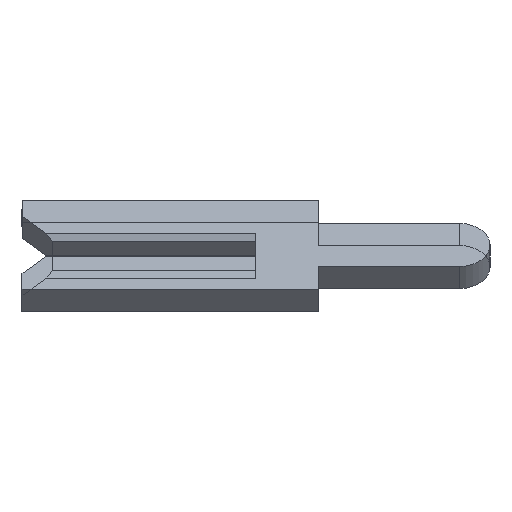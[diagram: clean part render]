
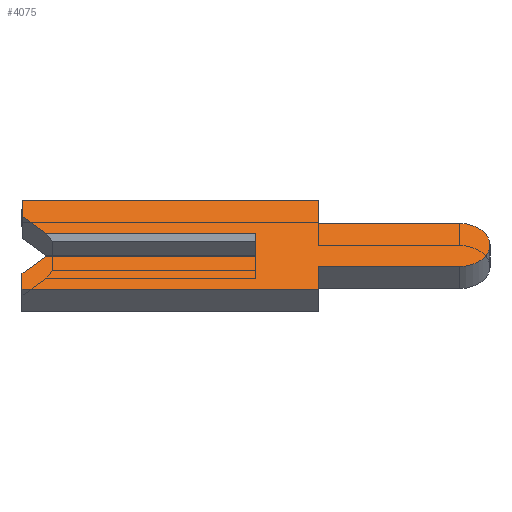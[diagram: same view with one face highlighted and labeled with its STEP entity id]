
A CAD part, left-side view. The second image highlights one B-rep face of the part: STEP entity #4075.
In plain terms, the highlighted face is planar.
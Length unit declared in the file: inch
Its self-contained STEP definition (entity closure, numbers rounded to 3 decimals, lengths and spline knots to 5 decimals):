
#40 = ORIENTED_EDGE ( 'NONE', *, *, #2204, .F. ) ;
#51 = CARTESIAN_POINT ( 'NONE',  ( -0.01, 0., 0.01 ) ) ;
#64 = CARTESIAN_POINT ( 'NONE',  ( -0.01, -0.04, 0.04 ) ) ;
#90 = LINE ( 'NONE', #1590, #3941 ) ;
#174 = VECTOR ( 'NONE', #2166, 39.37008 ) ;
#200 = LINE ( 'NONE', #1992, #308 ) ;
#203 = VERTEX_POINT ( 'NONE', #4058 ) ;
#227 = LINE ( 'NONE', #1441, #3796 ) ;
#308 = VECTOR ( 'NONE', #2768, 39.37008 ) ;
#315 = EDGE_CURVE ( 'NONE', #1802, #699, #2897, .T. ) ;
#431 = CARTESIAN_POINT ( 'NONE',  ( -0.01, 0.15, 0.04 ) ) ;
#466 = EDGE_CURVE ( 'NONE', #2783, #3046, #90, .T. ) ;
#490 = ORIENTED_EDGE ( 'NONE', *, *, #4316, .F. ) ;
#614 = LINE ( 'NONE', #3874, #3076 ) ;
#619 = CARTESIAN_POINT ( 'NONE',  ( -0.01, -0.1305, -0.0195 ) ) ;
#634 = DIRECTION ( 'NONE',  ( 0., 0., -1. ) ) ;
#636 = VERTEX_POINT ( 'NONE', #2024 ) ;
#690 = CARTESIAN_POINT ( 'NONE',  ( -0.01, 0.15, 0.04 ) ) ;
#695 = ORIENTED_EDGE ( 'NONE', *, *, #466, .F. ) ;
#699 = VERTEX_POINT ( 'NONE', #619 ) ;
#790 = PLANE ( 'NONE',  #916 ) ;
#916 = AXIS2_PLACEMENT_3D ( 'NONE', #3235, #1152, #1467 ) ;
#924 = LINE ( 'NONE', #3522, #949 ) ;
#929 = EDGE_LOOP ( 'NONE', ( #932, #3387, #4383, #3278, #1319, #1087, #40, #2142, #2138, #490, #3675, #3049, #695, #1218 ) ) ;
#932 = ORIENTED_EDGE ( 'NONE', *, *, #1268, .T. ) ;
#948 = VECTOR ( 'NONE', #4380, 39.37008 ) ;
#949 = VECTOR ( 'NONE', #2817, 39.37008 ) ;
#1085 = DIRECTION ( 'NONE',  ( 0., 0., 1. ) ) ;
#1087 = ORIENTED_EDGE ( 'NONE', *, *, #1785, .F. ) ;
#1152 = DIRECTION ( 'NONE',  ( 1., 0., 0. ) ) ;
#1169 = CARTESIAN_POINT ( 'NONE',  ( -0.01, -0.04, 0.0195 ) ) ;
#1218 = ORIENTED_EDGE ( 'NONE', *, *, #3611, .F. ) ;
#1268 = EDGE_CURVE ( 'NONE', #3727, #2309, #200, .T. ) ;
#1285 = LINE ( 'NONE', #431, #1708 ) ;
#1289 = LINE ( 'NONE', #4321, #2749 ) ;
#1319 = ORIENTED_EDGE ( 'NONE', *, *, #2436, .F. ) ;
#1441 = CARTESIAN_POINT ( 'NONE',  ( -0.01, 0.1305, -0.0065 ) ) ;
#1454 = CARTESIAN_POINT ( 'NONE',  ( -0.01, -0.04, -0.04 ) ) ;
#1467 = DIRECTION ( 'NONE',  ( 0., 0., -1. ) ) ;
#1501 = EDGE_CURVE ( 'NONE', #4048, #3283, #924, .T. ) ;
#1504 = LINE ( 'NONE', #1738, #3246 ) ;
#1590 = CARTESIAN_POINT ( 'NONE',  ( -0.01, 0.15, 0.026 ) ) ;
#1708 = VECTOR ( 'NONE', #4334, 39.37008 ) ;
#1738 = CARTESIAN_POINT ( 'NONE',  ( -0.01, 0., 0.0065 ) ) ;
#1761 = LINE ( 'NONE', #1916, #948 ) ;
#1767 = LINE ( 'NONE', #1454, #174 ) ;
#1785 = EDGE_CURVE ( 'NONE', #2020, #636, #614, .T. ) ;
#1801 = DIRECTION ( 'NONE',  ( 0., 0., 1. ) ) ;
#1802 = VERTEX_POINT ( 'NONE', #4162 ) ;
#1916 = CARTESIAN_POINT ( 'NONE',  ( -0.01, -0.04, 0.04 ) ) ;
#1943 = VECTOR ( 'NONE', #1801, 39.37008 ) ;
#1953 = DIRECTION ( 'NONE',  ( 0., 0., 1. ) ) ;
#1992 = CARTESIAN_POINT ( 'NONE',  ( -0.01, 0.15, 0.01 ) ) ;
#2020 = VERTEX_POINT ( 'NONE', #3491 ) ;
#2024 = CARTESIAN_POINT ( 'NONE',  ( -0.01, 0.15, -0.04 ) ) ;
#2107 = VECTOR ( 'NONE', #3654, 39.37008 ) ;
#2138 = ORIENTED_EDGE ( 'NONE', *, *, #315, .F. ) ;
#2142 = ORIENTED_EDGE ( 'NONE', *, *, #3190, .F. ) ;
#2166 = DIRECTION ( 'NONE',  ( 0., 0., -1. ) ) ;
#2192 = CARTESIAN_POINT ( 'NONE',  ( -0.01, 0.134, 0.01 ) ) ;
#2204 = EDGE_CURVE ( 'NONE', #2622, #2020, #1767, .T. ) ;
#2267 = EDGE_CURVE ( 'NONE', #203, #4048, #227, .T. ) ;
#2309 = VERTEX_POINT ( 'NONE', #51 ) ;
#2325 = LINE ( 'NONE', #1169, #2107 ) ;
#2328 = LINE ( 'NONE', #3498, #4070 ) ;
#2436 = EDGE_CURVE ( 'NONE', #636, #203, #2865, .T. ) ;
#2622 = VERTEX_POINT ( 'NONE', #3536 ) ;
#2680 = DIRECTION ( 'NONE',  ( 1., 0., 0. ) ) ;
#2749 = VECTOR ( 'NONE', #3256, 39.37008 ) ;
#2768 = DIRECTION ( 'NONE',  ( 0., -1., 0. ) ) ;
#2783 = VERTEX_POINT ( 'NONE', #4256 ) ;
#2817 = DIRECTION ( 'NONE',  ( 0., -1., 0. ) ) ;
#2865 = LINE ( 'NONE', #3537, #1943 ) ;
#2897 = CIRCLE ( 'NONE', #3096, 0.0195 ) ;
#3038 = EDGE_CURVE ( 'NONE', #3283, #2309, #1504, .T. ) ;
#3046 = VERTEX_POINT ( 'NONE', #690 ) ;
#3049 = ORIENTED_EDGE ( 'NONE', *, *, #3996, .F. ) ;
#3076 = VECTOR ( 'NONE', #3132, 39.37008 ) ;
#3096 = AXIS2_PLACEMENT_3D ( 'NONE', #4103, #2680, #634 ) ;
#3132 = DIRECTION ( 'NONE',  ( 0., 1., 0. ) ) ;
#3190 = EDGE_CURVE ( 'NONE', #699, #2622, #2328, .T. ) ;
#3220 = CARTESIAN_POINT ( 'NONE',  ( -0.01, 0.134, -0.01 ) ) ;
#3235 = CARTESIAN_POINT ( 'NONE',  ( -0.01, -0.1305, 0. ) ) ;
#3246 = VECTOR ( 'NONE', #1085, 39.37008 ) ;
#3256 = DIRECTION ( 'NONE',  ( 0., 0.707, 0.707 ) ) ;
#3278 = ORIENTED_EDGE ( 'NONE', *, *, #2267, .F. ) ;
#3283 = VERTEX_POINT ( 'NONE', #3903 ) ;
#3301 = CARTESIAN_POINT ( 'NONE',  ( -0.01, -0.04, 0.0195 ) ) ;
#3387 = ORIENTED_EDGE ( 'NONE', *, *, #3038, .F. ) ;
#3491 = CARTESIAN_POINT ( 'NONE',  ( -0.01, -0.04, -0.04 ) ) ;
#3498 = CARTESIAN_POINT ( 'NONE',  ( -0.01, -0.04, -0.0195 ) ) ;
#3522 = CARTESIAN_POINT ( 'NONE',  ( -0.01, -0.1305, -0.01 ) ) ;
#3536 = CARTESIAN_POINT ( 'NONE',  ( -0.01, -0.04, -0.0195 ) ) ;
#3537 = CARTESIAN_POINT ( 'NONE',  ( -0.01, 0.15, -0.026 ) ) ;
#3611 = EDGE_CURVE ( 'NONE', #3727, #2783, #1289, .T. ) ;
#3654 = DIRECTION ( 'NONE',  ( 0., -1., 0. ) ) ;
#3675 = ORIENTED_EDGE ( 'NONE', *, *, #4427, .F. ) ;
#3727 = VERTEX_POINT ( 'NONE', #2192 ) ;
#3796 = VECTOR ( 'NONE', #4279, 39.37008 ) ;
#3874 = CARTESIAN_POINT ( 'NONE',  ( -0.01, 0.15, -0.04 ) ) ;
#3903 = CARTESIAN_POINT ( 'NONE',  ( -0.01, 0., -0.01 ) ) ;
#3941 = VECTOR ( 'NONE', #1953, 39.37008 ) ;
#3947 = VERTEX_POINT ( 'NONE', #64 ) ;
#3996 = EDGE_CURVE ( 'NONE', #3046, #3947, #1285, .T. ) ;
#4048 = VERTEX_POINT ( 'NONE', #3220 ) ;
#4058 = CARTESIAN_POINT ( 'NONE',  ( -0.01, 0.15, -0.026 ) ) ;
#4070 = VECTOR ( 'NONE', #4203, 39.37008 ) ;
#4075 = ADVANCED_FACE ( 'NONE', ( #4399 ), #790, .F. ) ;
#4103 = CARTESIAN_POINT ( 'NONE',  ( -0.01, -0.1305, 0. ) ) ;
#4162 = CARTESIAN_POINT ( 'NONE',  ( -0.01, -0.1305, 0.0195 ) ) ;
#4203 = DIRECTION ( 'NONE',  ( 0., 1., 0. ) ) ;
#4256 = CARTESIAN_POINT ( 'NONE',  ( -0.01, 0.15, 0.026 ) ) ;
#4279 = DIRECTION ( 'NONE',  ( 0., -0.707, 0.707 ) ) ;
#4316 = EDGE_CURVE ( 'NONE', #4378, #1802, #2325, .T. ) ;
#4321 = CARTESIAN_POINT ( 'NONE',  ( -0.01, 0.1305, 0.0065 ) ) ;
#4334 = DIRECTION ( 'NONE',  ( 0., -1., 0. ) ) ;
#4378 = VERTEX_POINT ( 'NONE', #3301 ) ;
#4380 = DIRECTION ( 'NONE',  ( 0., 0., -1. ) ) ;
#4383 = ORIENTED_EDGE ( 'NONE', *, *, #1501, .F. ) ;
#4399 = FACE_OUTER_BOUND ( 'NONE', #929, .T. ) ;
#4427 = EDGE_CURVE ( 'NONE', #3947, #4378, #1761, .T. ) ;
